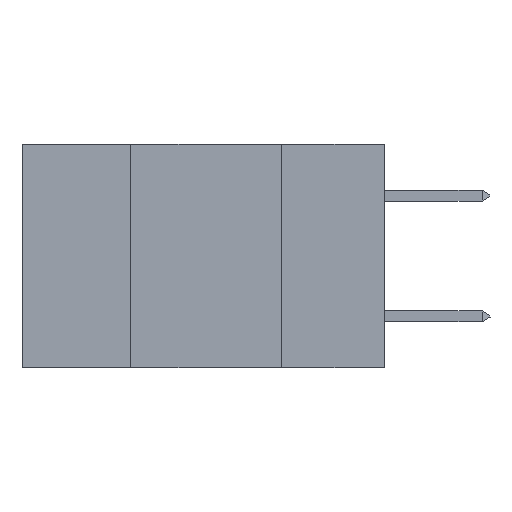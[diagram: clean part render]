
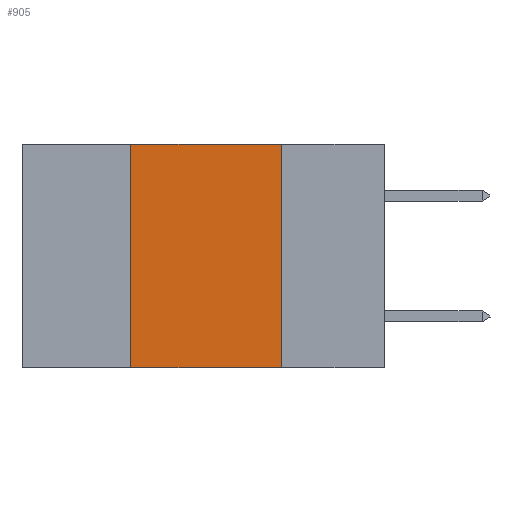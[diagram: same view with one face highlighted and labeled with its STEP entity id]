
A CAD part, left-side view. The second image highlights one B-rep face of the part: STEP entity #905.
In plain terms, the highlighted planar face has unit normal (-1, 0, 0).
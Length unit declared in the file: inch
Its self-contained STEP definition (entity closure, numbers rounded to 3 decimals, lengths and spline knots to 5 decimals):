
#814 = CARTESIAN_POINT ( 'NONE',  ( 0., 0.6, -0.37 ) ) ;
#905 = ADVANCED_FACE ( 'NONE', ( #20301 ), #17814, .F. ) ;
#1833 = CARTESIAN_POINT ( 'NONE',  ( 0., 0.17, 0. ) ) ;
#2194 = LINE ( 'NONE', #814, #3220 ) ;
#2682 = CARTESIAN_POINT ( 'NONE',  ( 0., 0.17, 0. ) ) ;
#2920 = LINE ( 'NONE', #11842, #13335 ) ;
#2957 = EDGE_LOOP ( 'NONE', ( #8835, #8760, #19673, #12270 ) ) ;
#3170 = DIRECTION ( 'NONE',  ( 1., 0., 0. ) ) ;
#3220 = VECTOR ( 'NONE', #11806, 39.37008 ) ;
#4113 = CARTESIAN_POINT ( 'NONE',  ( 0., 0.42, 0. ) ) ;
#4758 = VERTEX_POINT ( 'NONE', #13812 ) ;
#5636 = CARTESIAN_POINT ( 'NONE',  ( 0., 0.17, -0.37 ) ) ;
#6285 = EDGE_CURVE ( 'NONE', #4758, #7813, #27903, .T. ) ;
#7611 = EDGE_CURVE ( 'NONE', #4758, #22912, #2194, .T. ) ;
#7813 = VERTEX_POINT ( 'NONE', #21034 ) ;
#8760 = ORIENTED_EDGE ( 'NONE', *, *, #26511, .F. ) ;
#8765 = VECTOR ( 'NONE', #19138, 39.37008 ) ;
#8835 = ORIENTED_EDGE ( 'NONE', *, *, #24628, .F. ) ;
#11793 = AXIS2_PLACEMENT_3D ( 'NONE', #24615, #3170, #20036 ) ;
#11806 = DIRECTION ( 'NONE',  ( 0., -1., 0. ) ) ;
#11842 = CARTESIAN_POINT ( 'NONE',  ( 0., 0.6, 0. ) ) ;
#12270 = ORIENTED_EDGE ( 'NONE', *, *, #7611, .T. ) ;
#13335 = VECTOR ( 'NONE', #22386, 39.37008 ) ;
#13812 = CARTESIAN_POINT ( 'NONE',  ( 0., 0.42, -0.37 ) ) ;
#17814 = PLANE ( 'NONE',  #11793 ) ;
#19138 = DIRECTION ( 'NONE',  ( 0., 0., -1. ) ) ;
#19437 = DIRECTION ( 'NONE',  ( 0., 0., 1. ) ) ;
#19673 = ORIENTED_EDGE ( 'NONE', *, *, #6285, .F. ) ;
#20036 = DIRECTION ( 'NONE',  ( 0., 0., -1. ) ) ;
#20301 = FACE_OUTER_BOUND ( 'NONE', #2957, .T. ) ;
#20811 = VERTEX_POINT ( 'NONE', #2682 ) ;
#21034 = CARTESIAN_POINT ( 'NONE',  ( 0., 0.42, 0. ) ) ;
#21880 = LINE ( 'NONE', #1833, #8765 ) ;
#22386 = DIRECTION ( 'NONE',  ( 0., -1., 0. ) ) ;
#22823 = VECTOR ( 'NONE', #19437, 39.37008 ) ;
#22912 = VERTEX_POINT ( 'NONE', #5636 ) ;
#24615 = CARTESIAN_POINT ( 'NONE',  ( 0., 0.6, 0. ) ) ;
#24628 = EDGE_CURVE ( 'NONE', #20811, #22912, #21880, .T. ) ;
#26511 = EDGE_CURVE ( 'NONE', #7813, #20811, #2920, .T. ) ;
#27903 = LINE ( 'NONE', #4113, #22823 ) ;
